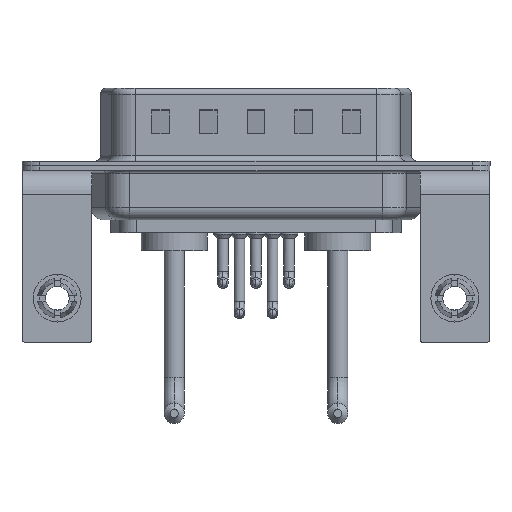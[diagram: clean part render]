
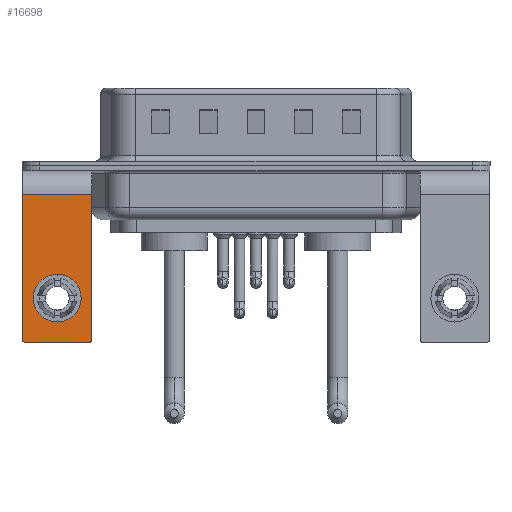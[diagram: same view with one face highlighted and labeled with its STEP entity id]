
A CAD part, front view. The second image highlights one B-rep face of the part: STEP entity #16698.
In plain terms, the highlighted planar face has unit normal (0, -1, 0).
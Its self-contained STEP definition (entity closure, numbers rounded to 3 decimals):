
#504 = DIRECTION ( 'NONE',  ( 0., -1., 0. ) ) ;
#907 = ORIENTED_EDGE ( 'NONE', *, *, #13549, .T. ) ;
#1467 = LINE ( 'NONE', #16173, #7192 ) ;
#1858 = ORIENTED_EDGE ( 'NONE', *, *, #14360, .T. ) ;
#2013 = VERTEX_POINT ( 'NONE', #11114 ) ;
#3215 = VERTEX_POINT ( 'NONE', #10433 ) ;
#3786 = CARTESIAN_POINT ( 'NONE',  ( 2.65, -6.25, -14.8 ) ) ;
#3989 = DIRECTION ( 'NONE',  ( 0., -1., 0. ) ) ;
#4385 = CARTESIAN_POINT ( 'NONE',  ( 2.9, -6.25, -14.55 ) ) ;
#4546 = CARTESIAN_POINT ( 'NONE',  ( 0., -6.25, -11.07 ) ) ;
#5307 = CIRCLE ( 'NONE', #10573, 0.25 ) ;
#6149 = EDGE_CURVE ( 'NONE', #13330, #11053, #9492, .T. ) ;
#6505 = LINE ( 'NONE', #22789, #7404 ) ;
#6541 = ORIENTED_EDGE ( 'NONE', *, *, #6149, .F. ) ;
#6871 = DIRECTION ( 'NONE',  ( 0., 0., 1. ) ) ;
#7114 = DIRECTION ( 'NONE',  ( 0., 1., 0. ) ) ;
#7192 = VECTOR ( 'NONE', #8536, 1000. ) ;
#7404 = VECTOR ( 'NONE', #19003, 1000. ) ;
#7672 = CARTESIAN_POINT ( 'NONE',  ( 2.65, -6.25, -14.55 ) ) ;
#7772 = VERTEX_POINT ( 'NONE', #15622 ) ;
#7993 = AXIS2_PLACEMENT_3D ( 'NONE', #18387, #3989, #16843 ) ;
#8536 = DIRECTION ( 'NONE',  ( 0., 0., -1. ) ) ;
#8675 = VERTEX_POINT ( 'NONE', #18597 ) ;
#8676 = AXIS2_PLACEMENT_3D ( 'NONE', #4546, #21072, #22839 ) ;
#9036 = CIRCLE ( 'NONE', #8676, 2. ) ;
#9335 = DIRECTION ( 'NONE',  ( 0., 0., 1. ) ) ;
#9492 = LINE ( 'NONE', #18359, #19742 ) ;
#10064 = CARTESIAN_POINT ( 'NONE',  ( -2.65, -6.25, -14.8 ) ) ;
#10433 = CARTESIAN_POINT ( 'NONE',  ( 2.9, -6.25, -2.4 ) ) ;
#10573 = AXIS2_PLACEMENT_3D ( 'NONE', #7672, #504, #9335 ) ;
#10644 = PLANE ( 'NONE',  #14201 ) ;
#10754 = DIRECTION ( 'NONE',  ( 0., 0., 1. ) ) ;
#10986 = FACE_OUTER_BOUND ( 'NONE', #18128, .T. ) ;
#11053 = VERTEX_POINT ( 'NONE', #10064 ) ;
#11114 = CARTESIAN_POINT ( 'NONE',  ( 0., -6.25, -13.07 ) ) ;
#11328 = EDGE_CURVE ( 'NONE', #7772, #14619, #1467, .T. ) ;
#11414 = EDGE_CURVE ( 'NONE', #13330, #17183, #5307, .T. ) ;
#12149 = DIRECTION ( 'NONE',  ( -1., 0., 0. ) ) ;
#13057 = EDGE_LOOP ( 'NONE', ( #17685, #1858 ) ) ;
#13330 = VERTEX_POINT ( 'NONE', #3786 ) ;
#13419 = ORIENTED_EDGE ( 'NONE', *, *, #11328, .T. ) ;
#13549 = EDGE_CURVE ( 'NONE', #3215, #7772, #17094, .T. ) ;
#13798 = EDGE_CURVE ( 'NONE', #14619, #11053, #14033, .T. ) ;
#14033 = CIRCLE ( 'NONE', #7993, 0.25 ) ;
#14174 = CIRCLE ( 'NONE', #14555, 2. ) ;
#14201 = AXIS2_PLACEMENT_3D ( 'NONE', #19732, #7114, #10754 ) ;
#14360 = EDGE_CURVE ( 'NONE', #8675, #2013, #9036, .T. ) ;
#14555 = AXIS2_PLACEMENT_3D ( 'NONE', #19725, #17482, #6871 ) ;
#14619 = VERTEX_POINT ( 'NONE', #19404 ) ;
#15407 = ORIENTED_EDGE ( 'NONE', *, *, #11414, .T. ) ;
#15622 = CARTESIAN_POINT ( 'NONE',  ( -2.9, -6.25, -2.4 ) ) ;
#15760 = ORIENTED_EDGE ( 'NONE', *, *, #18581, .F. ) ;
#16066 = FACE_BOUND ( 'NONE', #13057, .T. ) ;
#16173 = CARTESIAN_POINT ( 'NONE',  ( -2.9, -6.25, -2.4 ) ) ;
#16698 = ADVANCED_FACE ( 'NONE', ( #16066, #10986 ), #10644, .F. ) ;
#16843 = DIRECTION ( 'NONE',  ( 0., 0., 1. ) ) ;
#17094 = LINE ( 'NONE', #19116, #21567 ) ;
#17183 = VERTEX_POINT ( 'NONE', #4385 ) ;
#17482 = DIRECTION ( 'NONE',  ( 0., 1., 0. ) ) ;
#17685 = ORIENTED_EDGE ( 'NONE', *, *, #21465, .T. ) ;
#18128 = EDGE_LOOP ( 'NONE', ( #13419, #22759, #6541, #15407, #15760, #907 ) ) ;
#18359 = CARTESIAN_POINT ( 'NONE',  ( 2.9, -6.25, -14.8 ) ) ;
#18387 = CARTESIAN_POINT ( 'NONE',  ( -2.65, -6.25, -14.55 ) ) ;
#18581 = EDGE_CURVE ( 'NONE', #3215, #17183, #6505, .T. ) ;
#18597 = CARTESIAN_POINT ( 'NONE',  ( 0., -6.25, -9.07 ) ) ;
#19003 = DIRECTION ( 'NONE',  ( 0., 0., -1. ) ) ;
#19116 = CARTESIAN_POINT ( 'NONE',  ( 2.9, -6.25, -2.4 ) ) ;
#19404 = CARTESIAN_POINT ( 'NONE',  ( -2.9, -6.25, -14.55 ) ) ;
#19725 = CARTESIAN_POINT ( 'NONE',  ( 0., -6.25, -11.07 ) ) ;
#19732 = CARTESIAN_POINT ( 'NONE',  ( 2.9, -6.25, -2.4 ) ) ;
#19742 = VECTOR ( 'NONE', #19898, 1000. ) ;
#19898 = DIRECTION ( 'NONE',  ( -1., 0., 0. ) ) ;
#21072 = DIRECTION ( 'NONE',  ( 0., 1., 0. ) ) ;
#21465 = EDGE_CURVE ( 'NONE', #2013, #8675, #14174, .T. ) ;
#21567 = VECTOR ( 'NONE', #12149, 1000. ) ;
#22759 = ORIENTED_EDGE ( 'NONE', *, *, #13798, .T. ) ;
#22789 = CARTESIAN_POINT ( 'NONE',  ( 2.9, -6.25, -2.4 ) ) ;
#22839 = DIRECTION ( 'NONE',  ( 0., 0., 1. ) ) ;
